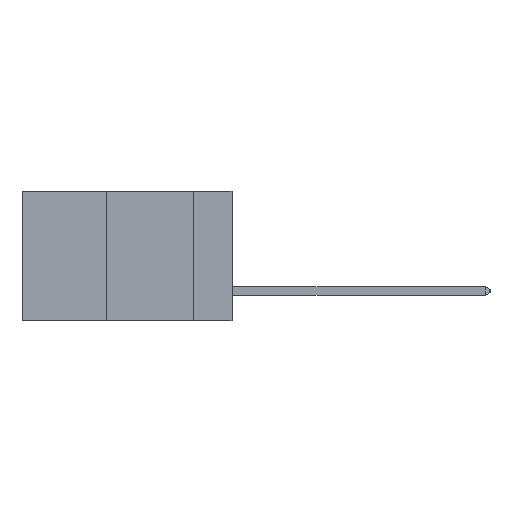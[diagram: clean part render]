
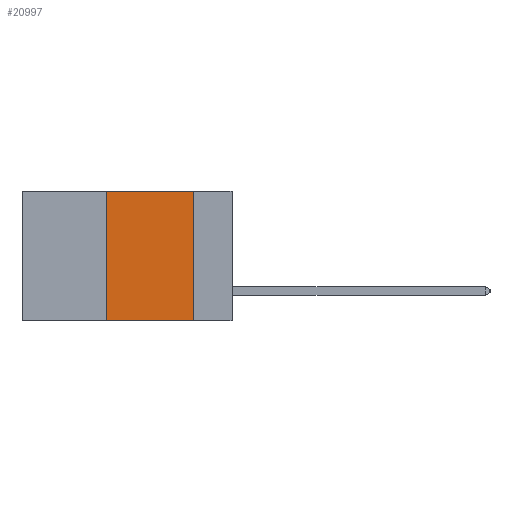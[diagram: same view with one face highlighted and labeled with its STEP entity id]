
A CAD part, left-side view. The second image highlights one B-rep face of the part: STEP entity #20997.
In plain terms, the highlighted planar face has unit normal (-1, 0, 0).
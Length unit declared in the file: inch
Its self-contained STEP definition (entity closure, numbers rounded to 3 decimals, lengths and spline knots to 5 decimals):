
#1073 = AXIS2_PLACEMENT_3D ( 'NONE', #10980, #12800, #2033 ) ;
#1202 = ORIENTED_EDGE ( 'NONE', *, *, #20366, .F. ) ;
#1663 = CARTESIAN_POINT ( 'NONE',  ( 0., 0.11, 0. ) ) ;
#2033 = DIRECTION ( 'NONE',  ( 0., 0., -1. ) ) ;
#2606 = EDGE_CURVE ( 'NONE', #20787, #18218, #14968, .T. ) ;
#2891 = ORIENTED_EDGE ( 'NONE', *, *, #2606, .F. ) ;
#3389 = LINE ( 'NONE', #8366, #12398 ) ;
#4752 = DIRECTION ( 'NONE',  ( 0., -1., 0. ) ) ;
#5032 = VECTOR ( 'NONE', #19559, 39.37008 ) ;
#6170 = EDGE_LOOP ( 'NONE', ( #1202, #6561, #2891, #7688 ) ) ;
#6561 = ORIENTED_EDGE ( 'NONE', *, *, #19619, .F. ) ;
#7394 = PLANE ( 'NONE',  #1073 ) ;
#7556 = FACE_OUTER_BOUND ( 'NONE', #6170, .T. ) ;
#7688 = ORIENTED_EDGE ( 'NONE', *, *, #8785, .T. ) ;
#8366 = CARTESIAN_POINT ( 'NONE',  ( 0., 0.6, 0. ) ) ;
#8625 = CARTESIAN_POINT ( 'NONE',  ( 0., 0.6, -0.37 ) ) ;
#8785 = EDGE_CURVE ( 'NONE', #20787, #14196, #22451, .T. ) ;
#8858 = VECTOR ( 'NONE', #21053, 39.37008 ) ;
#9145 = VERTEX_POINT ( 'NONE', #13170 ) ;
#9799 = LINE ( 'NONE', #1663, #5032 ) ;
#10194 = VECTOR ( 'NONE', #18999, 39.37008 ) ;
#10980 = CARTESIAN_POINT ( 'NONE',  ( 0., 0.6, 0. ) ) ;
#11773 = CARTESIAN_POINT ( 'NONE',  ( 0., 0.36, -0.37 ) ) ;
#12186 = CARTESIAN_POINT ( 'NONE',  ( 0., 0.36, 0. ) ) ;
#12398 = VECTOR ( 'NONE', #4752, 39.37008 ) ;
#12800 = DIRECTION ( 'NONE',  ( 1., 0., 0. ) ) ;
#13170 = CARTESIAN_POINT ( 'NONE',  ( 0., 0.11, 0. ) ) ;
#14196 = VERTEX_POINT ( 'NONE', #21931 ) ;
#14968 = LINE ( 'NONE', #20763, #10194 ) ;
#18218 = VERTEX_POINT ( 'NONE', #12186 ) ;
#18999 = DIRECTION ( 'NONE',  ( 0., 0., 1. ) ) ;
#19559 = DIRECTION ( 'NONE',  ( 0., 0., -1. ) ) ;
#19619 = EDGE_CURVE ( 'NONE', #18218, #9145, #3389, .T. ) ;
#20366 = EDGE_CURVE ( 'NONE', #9145, #14196, #9799, .T. ) ;
#20763 = CARTESIAN_POINT ( 'NONE',  ( 0., 0.36, 0. ) ) ;
#20787 = VERTEX_POINT ( 'NONE', #11773 ) ;
#20997 = ADVANCED_FACE ( 'NONE', ( #7556 ), #7394, .F. ) ;
#21053 = DIRECTION ( 'NONE',  ( 0., -1., 0. ) ) ;
#21931 = CARTESIAN_POINT ( 'NONE',  ( 0., 0.11, -0.37 ) ) ;
#22451 = LINE ( 'NONE', #8625, #8858 ) ;
